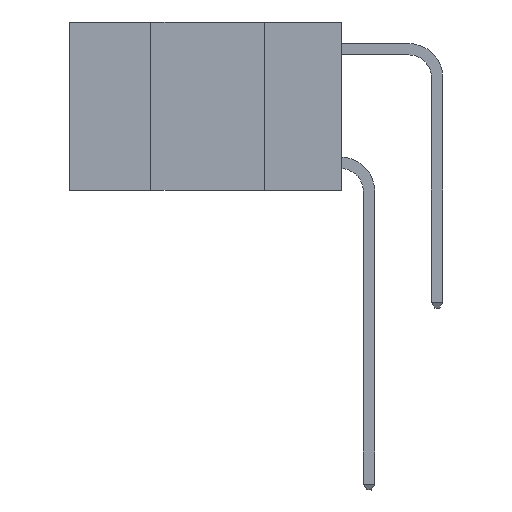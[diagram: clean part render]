
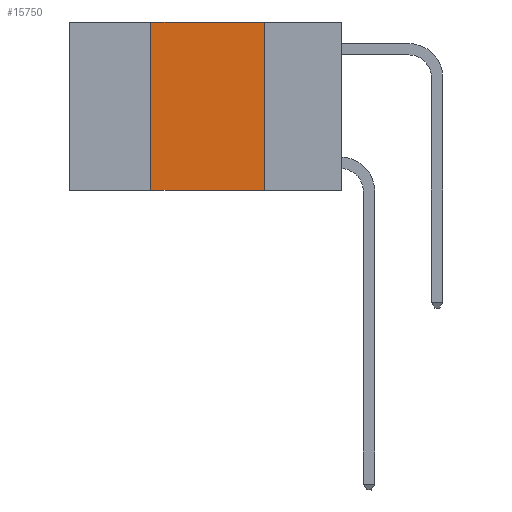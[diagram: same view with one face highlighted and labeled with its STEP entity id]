
A CAD part, left-side view. The second image highlights one B-rep face of the part: STEP entity #15750.
In plain terms, the highlighted planar face has unit normal (-1, 0, 0).
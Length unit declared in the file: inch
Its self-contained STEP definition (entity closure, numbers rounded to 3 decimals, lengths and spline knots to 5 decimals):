
#2161 = VECTOR ( 'NONE', #23387, 39.37008 ) ;
#2845 = VECTOR ( 'NONE', #29954, 39.37008 ) ;
#3099 = ORIENTED_EDGE ( 'NONE', *, *, #12758, .F. ) ;
#3824 = AXIS2_PLACEMENT_3D ( 'NONE', #22159, #13074, #29748 ) ;
#5383 = EDGE_CURVE ( 'NONE', #17321, #20635, #10180, .T. ) ;
#5701 = FACE_OUTER_BOUND ( 'NONE', #27860, .T. ) ;
#5897 = VERTEX_POINT ( 'NONE', #18459 ) ;
#6958 = VECTOR ( 'NONE', #28805, 39.37008 ) ;
#7918 = CARTESIAN_POINT ( 'NONE',  ( 0., 0.17, -0.37 ) ) ;
#7949 = ORIENTED_EDGE ( 'NONE', *, *, #12102, .F. ) ;
#10180 = LINE ( 'NONE', #24984, #28440 ) ;
#11368 = CARTESIAN_POINT ( 'NONE',  ( 0., 0.17, 0. ) ) ;
#12102 = EDGE_CURVE ( 'NONE', #13167, #5897, #26720, .T. ) ;
#12554 = PLANE ( 'NONE',  #3824 ) ;
#12758 = EDGE_CURVE ( 'NONE', #17321, #13167, #23753, .T. ) ;
#13074 = DIRECTION ( 'NONE',  ( 1., 0., 0. ) ) ;
#13167 = VERTEX_POINT ( 'NONE', #14784 ) ;
#14431 = CARTESIAN_POINT ( 'NONE',  ( 0., 0.42, 0. ) ) ;
#14784 = CARTESIAN_POINT ( 'NONE',  ( 0., 0.42, 0. ) ) ;
#15561 = CARTESIAN_POINT ( 'NONE',  ( 0., 0.42, -0.37 ) ) ;
#15750 = ADVANCED_FACE ( 'NONE', ( #5701 ), #12554, .F. ) ;
#17321 = VERTEX_POINT ( 'NONE', #15561 ) ;
#18459 = CARTESIAN_POINT ( 'NONE',  ( 0., 0.17, 0. ) ) ;
#20635 = VERTEX_POINT ( 'NONE', #7918 ) ;
#21071 = EDGE_CURVE ( 'NONE', #5897, #20635, #28660, .T. ) ;
#22159 = CARTESIAN_POINT ( 'NONE',  ( 0., 0.6, 0. ) ) ;
#23387 = DIRECTION ( 'NONE',  ( 0., 0., -1. ) ) ;
#23753 = LINE ( 'NONE', #14431, #6958 ) ;
#24984 = CARTESIAN_POINT ( 'NONE',  ( 0., 0.6, -0.37 ) ) ;
#26720 = LINE ( 'NONE', #29752, #2845 ) ;
#27190 = DIRECTION ( 'NONE',  ( 0., -1., 0. ) ) ;
#27855 = ORIENTED_EDGE ( 'NONE', *, *, #5383, .T. ) ;
#27860 = EDGE_LOOP ( 'NONE', ( #30120, #7949, #3099, #27855 ) ) ;
#28440 = VECTOR ( 'NONE', #27190, 39.37008 ) ;
#28660 = LINE ( 'NONE', #11368, #2161 ) ;
#28805 = DIRECTION ( 'NONE',  ( 0., 0., 1. ) ) ;
#29748 = DIRECTION ( 'NONE',  ( 0., 0., -1. ) ) ;
#29752 = CARTESIAN_POINT ( 'NONE',  ( 0., 0.6, 0. ) ) ;
#29954 = DIRECTION ( 'NONE',  ( 0., -1., 0. ) ) ;
#30120 = ORIENTED_EDGE ( 'NONE', *, *, #21071, .F. ) ;
